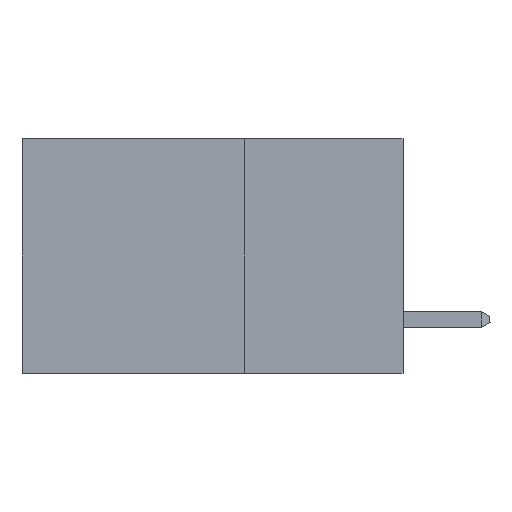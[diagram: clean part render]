
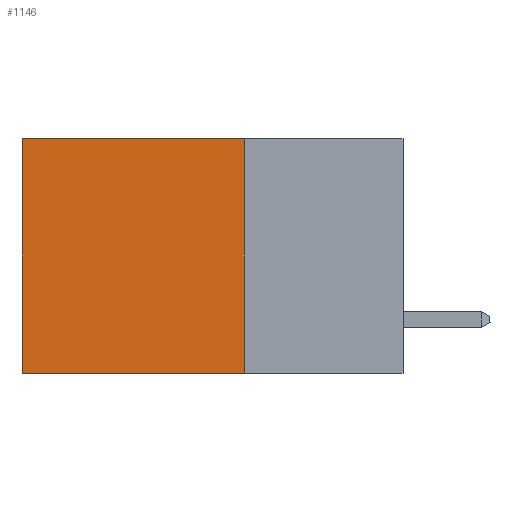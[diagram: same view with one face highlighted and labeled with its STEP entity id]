
A CAD part, left-side view. The second image highlights one B-rep face of the part: STEP entity #1146.
In plain terms, the highlighted planar face has unit normal (-1, 0, 0).
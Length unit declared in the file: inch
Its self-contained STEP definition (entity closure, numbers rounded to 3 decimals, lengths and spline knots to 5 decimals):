
#267 = EDGE_CURVE ( 'NONE', #4100, #1400, #555, .T. ) ;
#555 = LINE ( 'NONE', #10147, #2052 ) ;
#689 = LINE ( 'NONE', #5455, #5482 ) ;
#946 = EDGE_CURVE ( 'NONE', #4100, #2343, #8017, .T. ) ;
#1146 = ADVANCED_FACE ( 'NONE', ( #1565 ), #5785, .F. ) ;
#1400 = VERTEX_POINT ( 'NONE', #12173 ) ;
#1565 = FACE_OUTER_BOUND ( 'NONE', #12065, .T. ) ;
#1649 = ORIENTED_EDGE ( 'NONE', *, *, #946, .F. ) ;
#1849 = CARTESIAN_POINT ( 'NONE',  ( 0.2875, 0.25, -0.37 ) ) ;
#1940 = VERTEX_POINT ( 'NONE', #5585 ) ;
#2052 = VECTOR ( 'NONE', #3674, 39.37008 ) ;
#2343 = VERTEX_POINT ( 'NONE', #1849 ) ;
#3079 = VECTOR ( 'NONE', #5120, 39.37008 ) ;
#3266 = CARTESIAN_POINT ( 'NONE',  ( 0.2875, 0.25, 0. ) ) ;
#3674 = DIRECTION ( 'NONE',  ( 0., 1., 0. ) ) ;
#4100 = VERTEX_POINT ( 'NONE', #10365 ) ;
#4435 = EDGE_CURVE ( 'NONE', #1400, #1940, #11778, .T. ) ;
#4599 = ORIENTED_EDGE ( 'NONE', *, *, #11332, .F. ) ;
#4606 = ORIENTED_EDGE ( 'NONE', *, *, #267, .T. ) ;
#5120 = DIRECTION ( 'NONE',  ( 0., 0., -1. ) ) ;
#5153 = ORIENTED_EDGE ( 'NONE', *, *, #4435, .T. ) ;
#5455 = CARTESIAN_POINT ( 'NONE',  ( 0.2875, 0.25, -0.37 ) ) ;
#5482 = VECTOR ( 'NONE', #12252, 39.37008 ) ;
#5585 = CARTESIAN_POINT ( 'NONE',  ( 0.2875, 0.6, -0.37 ) ) ;
#5605 = CARTESIAN_POINT ( 'NONE',  ( 0.2875, 0.6, 0. ) ) ;
#5785 = PLANE ( 'NONE',  #6759 ) ;
#6759 = AXIS2_PLACEMENT_3D ( 'NONE', #3266, #6954, #8937 ) ;
#6954 = DIRECTION ( 'NONE',  ( 1., 0., 0. ) ) ;
#7445 = CARTESIAN_POINT ( 'NONE',  ( 0.2875, 0.25, 0. ) ) ;
#8017 = LINE ( 'NONE', #7445, #10576 ) ;
#8937 = DIRECTION ( 'NONE',  ( 0., 0., -1. ) ) ;
#10147 = CARTESIAN_POINT ( 'NONE',  ( 0.2875, 0.25, 0. ) ) ;
#10275 = DIRECTION ( 'NONE',  ( 0., 0., -1. ) ) ;
#10365 = CARTESIAN_POINT ( 'NONE',  ( 0.2875, 0.25, 0. ) ) ;
#10576 = VECTOR ( 'NONE', #10275, 39.37008 ) ;
#11332 = EDGE_CURVE ( 'NONE', #2343, #1940, #689, .T. ) ;
#11778 = LINE ( 'NONE', #5605, #3079 ) ;
#12065 = EDGE_LOOP ( 'NONE', ( #5153, #4599, #1649, #4606 ) ) ;
#12173 = CARTESIAN_POINT ( 'NONE',  ( 0.2875, 0.6, 0. ) ) ;
#12252 = DIRECTION ( 'NONE',  ( 0., 1., 0. ) ) ;
